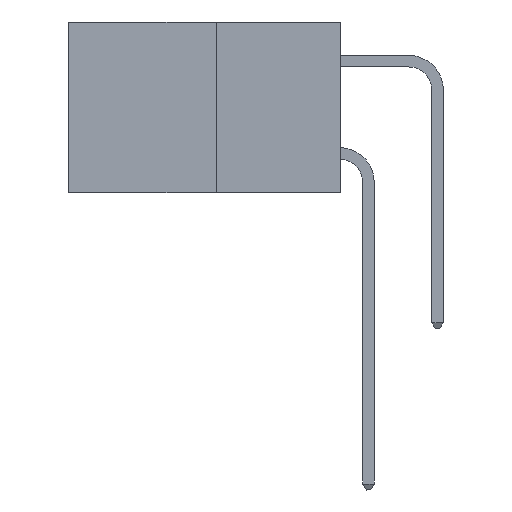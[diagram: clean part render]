
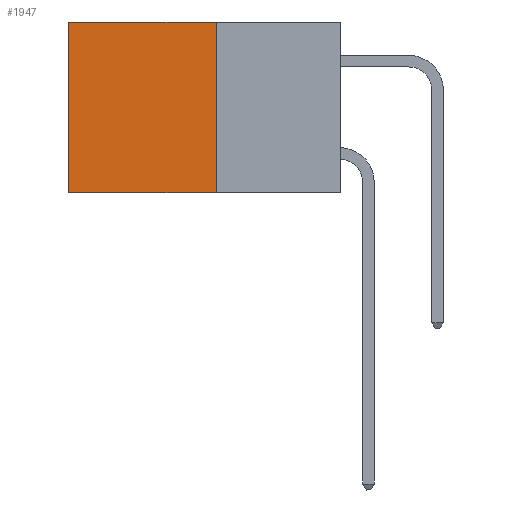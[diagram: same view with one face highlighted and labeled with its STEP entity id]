
A CAD part, left-side view. The second image highlights one B-rep face of the part: STEP entity #1947.
In plain terms, the highlighted planar face has unit normal (-1, 0, 0).
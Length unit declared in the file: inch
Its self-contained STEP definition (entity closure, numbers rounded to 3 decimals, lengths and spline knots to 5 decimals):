
#211 = VERTEX_POINT ( 'NONE', #4854 ) ;
#1139 = VERTEX_POINT ( 'NONE', #14103 ) ;
#1947 = ADVANCED_FACE ( 'NONE', ( #3538 ), #6752, .F. ) ;
#3538 = FACE_OUTER_BOUND ( 'NONE', #8752, .T. ) ;
#4776 = LINE ( 'NONE', #16282, #15421 ) ;
#4854 = CARTESIAN_POINT ( 'NONE',  ( 0.277, 0.59, 0. ) ) ;
#4935 = CARTESIAN_POINT ( 'NONE',  ( 0.277, 0.27, 0. ) ) ;
#5153 = LINE ( 'NONE', #9049, #9788 ) ;
#5471 = EDGE_CURVE ( 'NONE', #15084, #1139, #4776, .T. ) ;
#6197 = ORIENTED_EDGE ( 'NONE', *, *, #10007, .T. ) ;
#6331 = CARTESIAN_POINT ( 'NONE',  ( 0.277, 0.59, -0.37 ) ) ;
#6440 = CARTESIAN_POINT ( 'NONE',  ( 0.277, 0.27, -0.37 ) ) ;
#6752 = PLANE ( 'NONE',  #13800 ) ;
#6886 = LINE ( 'NONE', #6440, #17428 ) ;
#7496 = ORIENTED_EDGE ( 'NONE', *, *, #11135, .T. ) ;
#7846 = DIRECTION ( 'NONE',  ( 0., 1., 0. ) ) ;
#8752 = EDGE_LOOP ( 'NONE', ( #6197, #17176, #17609, #7496 ) ) ;
#9049 = CARTESIAN_POINT ( 'NONE',  ( 0.277, 0.27, 0. ) ) ;
#9607 = LINE ( 'NONE', #12398, #12027 ) ;
#9788 = VECTOR ( 'NONE', #10475, 39.37008 ) ;
#10007 = EDGE_CURVE ( 'NONE', #211, #18037, #9607, .T. ) ;
#10475 = DIRECTION ( 'NONE',  ( 0., 1., 0. ) ) ;
#10622 = DIRECTION ( 'NONE',  ( 1., 0., 0. ) ) ;
#11008 = DIRECTION ( 'NONE',  ( 0., 0., -1. ) ) ;
#11135 = EDGE_CURVE ( 'NONE', #15084, #211, #5153, .T. ) ;
#12027 = VECTOR ( 'NONE', #11008, 39.37008 ) ;
#12398 = CARTESIAN_POINT ( 'NONE',  ( 0.277, 0.59, -0.37 ) ) ;
#12530 = EDGE_CURVE ( 'NONE', #1139, #18037, #6886, .T. ) ;
#13800 = AXIS2_PLACEMENT_3D ( 'NONE', #15888, #10622, #17663 ) ;
#14103 = CARTESIAN_POINT ( 'NONE',  ( 0.277, 0.27, -0.37 ) ) ;
#14885 = DIRECTION ( 'NONE',  ( 0., 0., -1. ) ) ;
#15084 = VERTEX_POINT ( 'NONE', #4935 ) ;
#15421 = VECTOR ( 'NONE', #14885, 39.37008 ) ;
#15888 = CARTESIAN_POINT ( 'NONE',  ( 0.277, 0.27, -0.37 ) ) ;
#16282 = CARTESIAN_POINT ( 'NONE',  ( 0.277, 0.27, -0.37 ) ) ;
#17176 = ORIENTED_EDGE ( 'NONE', *, *, #12530, .F. ) ;
#17428 = VECTOR ( 'NONE', #7846, 39.37008 ) ;
#17609 = ORIENTED_EDGE ( 'NONE', *, *, #5471, .F. ) ;
#17663 = DIRECTION ( 'NONE',  ( 0., 0., -1. ) ) ;
#18037 = VERTEX_POINT ( 'NONE', #6331 ) ;
